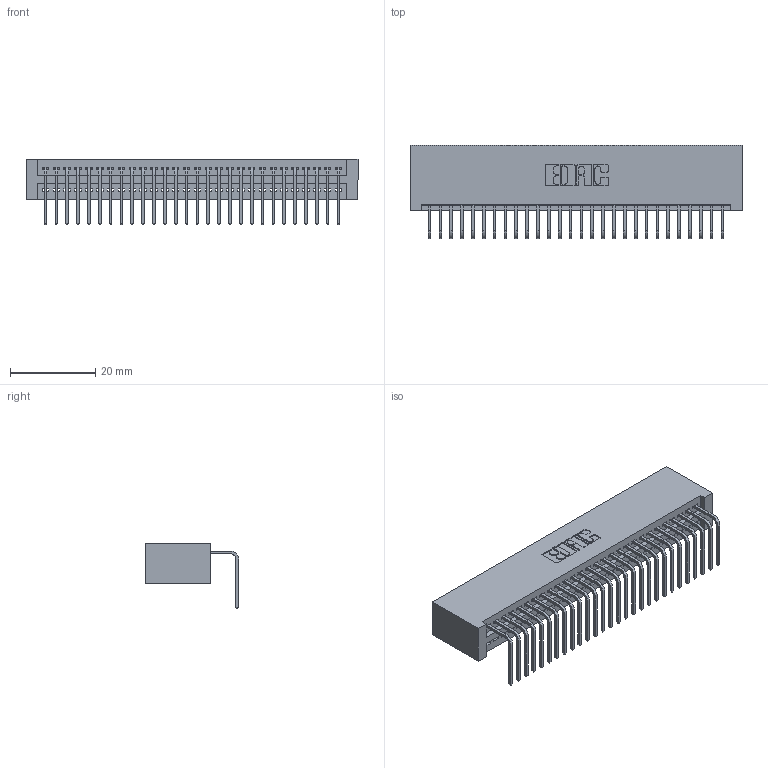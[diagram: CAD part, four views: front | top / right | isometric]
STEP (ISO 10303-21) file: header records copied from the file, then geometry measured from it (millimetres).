
FILE_DESCRIPTION (( 'STEP AP203' ), '1' );
FILE_NAME ('345-028-558-101.STEP', '2018-08-22T23:18:14', ( '' ), ( '' ), 'SwSTEP 2.0', 'SolidWorks 2016', '' );
FILE_SCHEMA (( 'CONFIG_CONTROL_DESIGN' ));
Length unit declared in the file: inch
Products named in the file (3): 345 Part_No Mounting Lugs; 345-292-001_558 Tail - 2; 345-028-558-101
Assembly tree (29 placements, depth 2):
  345-028-558-101
    345 Part_No Mounting Lugs
    345-292-001_558 Tail - 2  x28
Bounding box: 77.72 x 21.83 x 15.37 mm (x, y, z)
Volume: 7945.3 mm3; surface area: 11106.6 mm2
Topology: 29 solids, 29 shells, 1798 faces, 5413 edges, 3570 vertices
Faces by surface type: plane 1252, cylinder 546
Entity records: 22765 total; most frequent: CARTESIAN_POINT 3952, ORIENTED_EDGE 3914, DIRECTION 3465, EDGE_CURVE 1957, LINE 1721, VECTOR 1721, VERTEX_POINT 1302, AXIS2_PLACEMENT_3D 872
